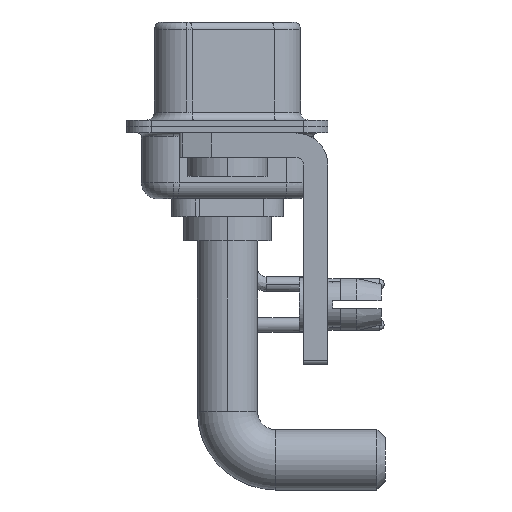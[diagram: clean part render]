
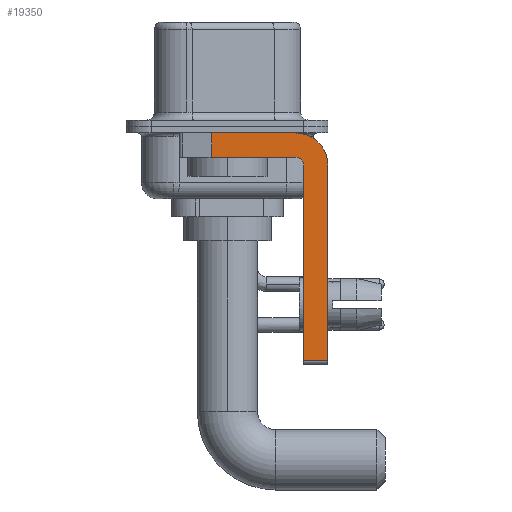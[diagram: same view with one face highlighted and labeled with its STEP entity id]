
A CAD part, left-side view. The second image highlights one B-rep face of the part: STEP entity #19350.
In plain terms, the highlighted planar face has unit normal (-1, 0, 0).
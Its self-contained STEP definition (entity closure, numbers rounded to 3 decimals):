
#361 = EDGE_CURVE ( 'NONE', #15637, #10828, #974, .T. ) ;
#974 = LINE ( 'NONE', #28156, #21065 ) ;
#1371 = PLANE ( 'NONE',  #10168 ) ;
#1570 = ORIENTED_EDGE ( 'NONE', *, *, #23848, .F. ) ;
#1605 = DIRECTION ( 'NONE',  ( 0., 0., -1. ) ) ;
#1731 = DIRECTION ( 'NONE',  ( 0., -1., 0. ) ) ;
#1779 = VERTEX_POINT ( 'NONE', #10474 ) ;
#2292 = EDGE_CURVE ( 'NONE', #12666, #1779, #28243, .T. ) ;
#2491 = ORIENTED_EDGE ( 'NONE', *, *, #18905, .F. ) ;
#2978 = ORIENTED_EDGE ( 'NONE', *, *, #13806, .T. ) ;
#3020 = VECTOR ( 'NONE', #1731, 1000. ) ;
#3736 = DIRECTION ( 'NONE',  ( 0., 0., -1. ) ) ;
#4177 = CARTESIAN_POINT ( 'NONE',  ( -2.9, 0.978, -1.9 ) ) ;
#5453 = ORIENTED_EDGE ( 'NONE', *, *, #22914, .F. ) ;
#5536 = DIRECTION ( 'NONE',  ( 0., 1., 0. ) ) ;
#5863 = DIRECTION ( 'NONE',  ( -1., 0., 0. ) ) ;
#6133 = EDGE_CURVE ( 'NONE', #25592, #22827, #10343, .T. ) ;
#7801 = DIRECTION ( 'NONE',  ( 0., 0., -1. ) ) ;
#8398 = CARTESIAN_POINT ( 'NONE',  ( -2.9, -4.25, -14.55 ) ) ;
#8566 = CARTESIAN_POINT ( 'NONE',  ( -2.9, -6.25, -2.4 ) ) ;
#9465 = CARTESIAN_POINT ( 'NONE',  ( -2.9, -4.75, -14.8 ) ) ;
#10063 = CARTESIAN_POINT ( 'NONE',  ( -2.9, -4.25, -0.4 ) ) ;
#10168 = AXIS2_PLACEMENT_3D ( 'NONE', #28538, #24074, #3736 ) ;
#10343 = LINE ( 'NONE', #15398, #17038 ) ;
#10474 = CARTESIAN_POINT ( 'NONE',  ( -2.9, -4.25, -1.9 ) ) ;
#10562 = EDGE_CURVE ( 'NONE', #1779, #10828, #12195, .T. ) ;
#10828 = VERTEX_POINT ( 'NONE', #4177 ) ;
#12195 = LINE ( 'NONE', #16806, #26655 ) ;
#12666 = VERTEX_POINT ( 'NONE', #16896 ) ;
#12690 = ORIENTED_EDGE ( 'NONE', *, *, #2292, .F. ) ;
#12692 = VERTEX_POINT ( 'NONE', #10063 ) ;
#12817 = CARTESIAN_POINT ( 'NONE',  ( -2.9, -4.25, -2.4 ) ) ;
#12994 = CIRCLE ( 'NONE', #18699, 2. ) ;
#13052 = AXIS2_PLACEMENT_3D ( 'NONE', #12817, #5863, #28731 ) ;
#13054 = ORIENTED_EDGE ( 'NONE', *, *, #6133, .F. ) ;
#13780 = CARTESIAN_POINT ( 'NONE',  ( -2.9, 3., -0.4 ) ) ;
#13802 = CARTESIAN_POINT ( 'NONE',  ( -2.9, 0.978, -0.4 ) ) ;
#13806 = EDGE_CURVE ( 'NONE', #28484, #22827, #21760, .T. ) ;
#15398 = CARTESIAN_POINT ( 'NONE',  ( -2.9, -6.25, -2.4 ) ) ;
#15637 = VERTEX_POINT ( 'NONE', #13802 ) ;
#15718 = DIRECTION ( 'NONE',  ( 0., -1., 0. ) ) ;
#16806 = CARTESIAN_POINT ( 'NONE',  ( -2.9, -4.25, -1.9 ) ) ;
#16896 = CARTESIAN_POINT ( 'NONE',  ( -2.9, -4.75, -2.4 ) ) ;
#17038 = VECTOR ( 'NONE', #1605, 1000. ) ;
#17825 = CARTESIAN_POINT ( 'NONE',  ( -2.9, -4.25, -2.4 ) ) ;
#18699 = AXIS2_PLACEMENT_3D ( 'NONE', #17825, #26890, #24208 ) ;
#18866 = VECTOR ( 'NONE', #27608, 1000. ) ;
#18905 = EDGE_CURVE ( 'NONE', #12692, #25592, #12994, .T. ) ;
#19350 = ADVANCED_FACE ( 'NONE', ( #23931 ), #1371, .F. ) ;
#19705 = CARTESIAN_POINT ( 'NONE',  ( -2.9, -4.75, -14.55 ) ) ;
#20761 = LINE ( 'NONE', #9465, #18866 ) ;
#20764 = LINE ( 'NONE', #13780, #20827 ) ;
#20827 = VECTOR ( 'NONE', #15718, 1000. ) ;
#20904 = CARTESIAN_POINT ( 'NONE',  ( -2.9, -6.25, -14.55 ) ) ;
#21065 = VECTOR ( 'NONE', #7801, 1000. ) ;
#21248 = ORIENTED_EDGE ( 'NONE', *, *, #10562, .F. ) ;
#21760 = LINE ( 'NONE', #8398, #3020 ) ;
#22827 = VERTEX_POINT ( 'NONE', #20904 ) ;
#22914 = EDGE_CURVE ( 'NONE', #28484, #12666, #20761, .T. ) ;
#23848 = EDGE_CURVE ( 'NONE', #15637, #12692, #20764, .T. ) ;
#23931 = FACE_OUTER_BOUND ( 'NONE', #25791, .T. ) ;
#24074 = DIRECTION ( 'NONE',  ( 1., 0., 0. ) ) ;
#24208 = DIRECTION ( 'NONE',  ( 0., 0., -1. ) ) ;
#25592 = VERTEX_POINT ( 'NONE', #8566 ) ;
#25791 = EDGE_LOOP ( 'NONE', ( #1570, #26418, #21248, #12690, #5453, #2978, #13054, #2491 ) ) ;
#26418 = ORIENTED_EDGE ( 'NONE', *, *, #361, .T. ) ;
#26655 = VECTOR ( 'NONE', #5536, 1000. ) ;
#26890 = DIRECTION ( 'NONE',  ( 1., 0., 0. ) ) ;
#27608 = DIRECTION ( 'NONE',  ( 0., 0., 1. ) ) ;
#28156 = CARTESIAN_POINT ( 'NONE',  ( -2.9, 0.978, -1.9 ) ) ;
#28243 = CIRCLE ( 'NONE', #13052, 0.5 ) ;
#28484 = VERTEX_POINT ( 'NONE', #19705 ) ;
#28538 = CARTESIAN_POINT ( 'NONE',  ( -2.9, -4.25, -2.4 ) ) ;
#28731 = DIRECTION ( 'NONE',  ( 0., 0., 1. ) ) ;
